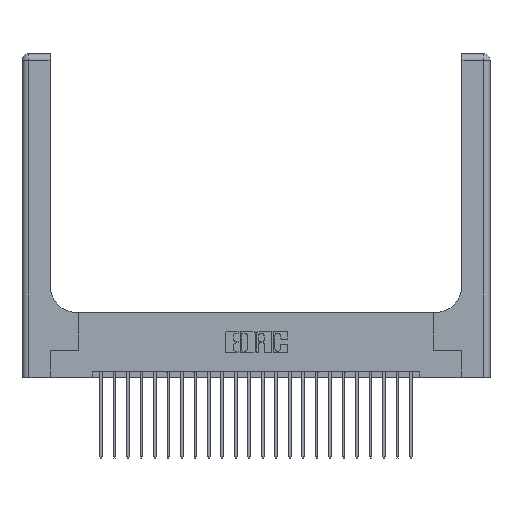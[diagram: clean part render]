
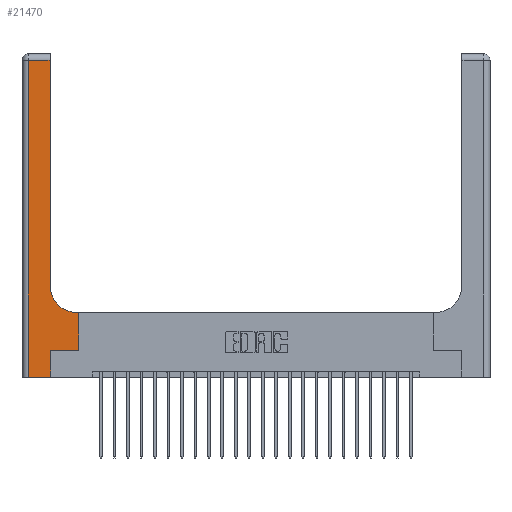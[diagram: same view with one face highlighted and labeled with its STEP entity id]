
A CAD part, top view. The second image highlights one B-rep face of the part: STEP entity #21470.
In plain terms, the highlighted planar face has unit normal (0, 0, 1).
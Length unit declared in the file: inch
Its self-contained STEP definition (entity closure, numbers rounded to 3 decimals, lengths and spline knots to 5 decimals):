
#258 = DIRECTION ( 'NONE',  ( 1., 0., 0. ) ) ;
#270 = EDGE_CURVE ( 'NONE', #11405, #16679, #11412, .T. ) ;
#401 = LINE ( 'NONE', #18786, #11048 ) ;
#428 = CARTESIAN_POINT ( 'NONE',  ( 0.06, 0., 0.37 ) ) ;
#674 = VECTOR ( 'NONE', #7346, 39.37008 ) ;
#815 = EDGE_CURVE ( 'NONE', #2908, #11470, #21124, .T. ) ;
#820 = VERTEX_POINT ( 'NONE', #4544 ) ;
#1575 = EDGE_CURVE ( 'NONE', #10978, #11405, #9754, .T. ) ;
#1672 = ORIENTED_EDGE ( 'NONE', *, *, #815, .T. ) ;
#1916 = DIRECTION ( 'NONE',  ( -1., 0., 0. ) ) ;
#2155 = CARTESIAN_POINT ( 'NONE',  ( 0., 2.94, 0.37 ) ) ;
#2392 = ORIENTED_EDGE ( 'NONE', *, *, #1575, .T. ) ;
#2432 = ORIENTED_EDGE ( 'NONE', *, *, #10497, .T. ) ;
#2680 = CARTESIAN_POINT ( 'NONE',  ( 0.528, 0.25, 0.37 ) ) ;
#2908 = VERTEX_POINT ( 'NONE', #2680 ) ;
#3470 = EDGE_CURVE ( 'NONE', #820, #2908, #19697, .T. ) ;
#4544 = CARTESIAN_POINT ( 'NONE',  ( 0.265, 0.25, 0.37 ) ) ;
#4546 = LINE ( 'NONE', #6547, #6838 ) ;
#4662 = DIRECTION ( 'NONE',  ( 0., 0., -1. ) ) ;
#4693 = CARTESIAN_POINT ( 'NONE',  ( 0.265, 0.25, 0.37 ) ) ;
#4761 = DIRECTION ( 'NONE',  ( -1., 0., 0. ) ) ;
#5344 = EDGE_LOOP ( 'NONE', ( #17892, #11773, #2392, #20367, #2432, #20150, #1672, #18112, #9041 ) ) ;
#5789 = DIRECTION ( 'NONE',  ( -1., 0., 0. ) ) ;
#5832 = VECTOR ( 'NONE', #1916, 39.37008 ) ;
#5861 = EDGE_CURVE ( 'NONE', #6663, #16188, #4546, .T. ) ;
#6082 = VERTEX_POINT ( 'NONE', #14130 ) ;
#6169 = CARTESIAN_POINT ( 'NONE',  ( 0.528, 0.6, 0.37 ) ) ;
#6547 = CARTESIAN_POINT ( 'NONE',  ( 0.26, 3., 0.37 ) ) ;
#6663 = VERTEX_POINT ( 'NONE', #13923 ) ;
#6838 = VECTOR ( 'NONE', #13892, 39.37008 ) ;
#7099 = LINE ( 'NONE', #13011, #674 ) ;
#7346 = DIRECTION ( 'NONE',  ( 0., 1., 0. ) ) ;
#7643 = CIRCLE ( 'NONE', #17230, 0.25 ) ;
#8688 = VECTOR ( 'NONE', #13929, 39.37008 ) ;
#9041 = ORIENTED_EDGE ( 'NONE', *, *, #18024, .T. ) ;
#9754 = LINE ( 'NONE', #15173, #15617 ) ;
#9818 = CARTESIAN_POINT ( 'NONE',  ( 0.528, 0.25, 0.37 ) ) ;
#9824 = PLANE ( 'NONE',  #13148 ) ;
#10063 = DIRECTION ( 'NONE',  ( 1., 0., 0. ) ) ;
#10308 = CARTESIAN_POINT ( 'NONE',  ( 0.51, 0.85, 0.37 ) ) ;
#10497 = EDGE_CURVE ( 'NONE', #16679, #820, #7099, .T. ) ;
#10978 = VERTEX_POINT ( 'NONE', #18473 ) ;
#11048 = VECTOR ( 'NONE', #5789, 39.37008 ) ;
#11168 = CARTESIAN_POINT ( 'NONE',  ( 0., 0., 0.37 ) ) ;
#11405 = VERTEX_POINT ( 'NONE', #428 ) ;
#11412 = LINE ( 'NONE', #11168, #19375 ) ;
#11470 = VERTEX_POINT ( 'NONE', #6169 ) ;
#11773 = ORIENTED_EDGE ( 'NONE', *, *, #21277, .T. ) ;
#11913 = DIRECTION ( 'NONE',  ( 0., -1., 0. ) ) ;
#13011 = CARTESIAN_POINT ( 'NONE',  ( 0.265, 0., 0.37 ) ) ;
#13148 = AXIS2_PLACEMENT_3D ( 'NONE', #15587, #4662, #4761 ) ;
#13430 = DIRECTION ( 'NONE',  ( 0., 1., 0. ) ) ;
#13892 = DIRECTION ( 'NONE',  ( 0., 1., 0. ) ) ;
#13923 = CARTESIAN_POINT ( 'NONE',  ( 0.26, 0.85, 0.37 ) ) ;
#13929 = DIRECTION ( 'NONE',  ( 1., 0., 0. ) ) ;
#14033 = DIRECTION ( 'NONE',  ( 0., 0., -1. ) ) ;
#14130 = CARTESIAN_POINT ( 'NONE',  ( 0.51, 0.6, 0.37 ) ) ;
#15173 = CARTESIAN_POINT ( 'NONE',  ( 0.06, 3., 0.37 ) ) ;
#15587 = CARTESIAN_POINT ( 'NONE',  ( 0., 3., 0.37 ) ) ;
#15617 = VECTOR ( 'NONE', #11913, 39.37008 ) ;
#16188 = VERTEX_POINT ( 'NONE', #16584 ) ;
#16584 = CARTESIAN_POINT ( 'NONE',  ( 0.26, 2.94, 0.37 ) ) ;
#16679 = VERTEX_POINT ( 'NONE', #19632 ) ;
#17230 = AXIS2_PLACEMENT_3D ( 'NONE', #10308, #14033, #10063 ) ;
#17466 = EDGE_CURVE ( 'NONE', #11470, #6082, #401, .T. ) ;
#17491 = VECTOR ( 'NONE', #13430, 39.37008 ) ;
#17892 = ORIENTED_EDGE ( 'NONE', *, *, #5861, .T. ) ;
#18024 = EDGE_CURVE ( 'NONE', #6082, #6663, #7643, .T. ) ;
#18112 = ORIENTED_EDGE ( 'NONE', *, *, #17466, .T. ) ;
#18473 = CARTESIAN_POINT ( 'NONE',  ( 0.06, 2.94, 0.37 ) ) ;
#18786 = CARTESIAN_POINT ( 'NONE',  ( 0.26, 0.6, 0.37 ) ) ;
#19375 = VECTOR ( 'NONE', #258, 39.37008 ) ;
#19632 = CARTESIAN_POINT ( 'NONE',  ( 0.265, 0., 0.37 ) ) ;
#19697 = LINE ( 'NONE', #4693, #8688 ) ;
#20150 = ORIENTED_EDGE ( 'NONE', *, *, #3470, .T. ) ;
#20367 = ORIENTED_EDGE ( 'NONE', *, *, #270, .T. ) ;
#21124 = LINE ( 'NONE', #9818, #17491 ) ;
#21277 = EDGE_CURVE ( 'NONE', #16188, #10978, #22452, .T. ) ;
#21470 = ADVANCED_FACE ( 'NONE', ( #23037 ), #9824, .F. ) ;
#22452 = LINE ( 'NONE', #2155, #5832 ) ;
#23037 = FACE_OUTER_BOUND ( 'NONE', #5344, .T. ) ;
